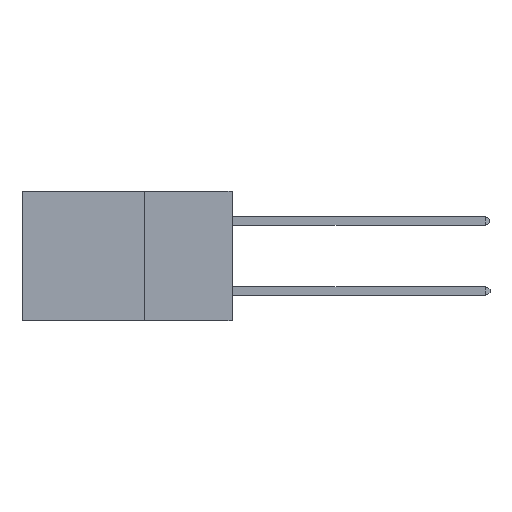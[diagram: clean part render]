
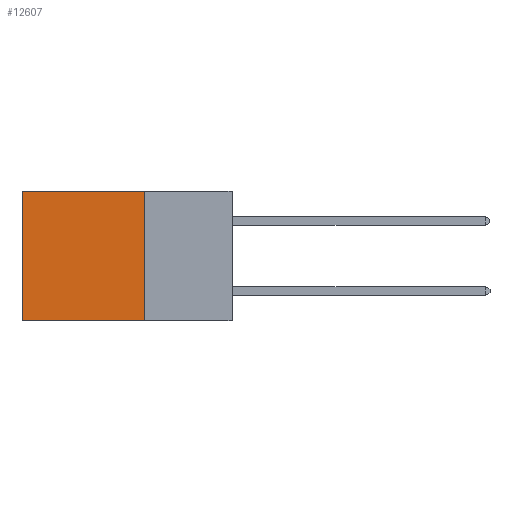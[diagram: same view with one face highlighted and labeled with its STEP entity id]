
A CAD part, left-side view. The second image highlights one B-rep face of the part: STEP entity #12607.
In plain terms, the highlighted planar face has unit normal (-1, 0, 0).
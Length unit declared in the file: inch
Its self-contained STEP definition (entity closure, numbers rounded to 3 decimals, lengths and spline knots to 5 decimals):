
#55 = ORIENTED_EDGE ( 'NONE', *, *, #5536, .T. ) ;
#754 = EDGE_CURVE ( 'NONE', #19839, #10343, #6532, .T. ) ;
#950 = CARTESIAN_POINT ( 'NONE',  ( 0.2875, 0.25, 0. ) ) ;
#1125 = DIRECTION ( 'NONE',  ( 0., 0., -1. ) ) ;
#1628 = VECTOR ( 'NONE', #1125, 39.37008 ) ;
#1685 = CARTESIAN_POINT ( 'NONE',  ( 0.2875, 0.6, 0. ) ) ;
#2611 = LINE ( 'NONE', #9584, #20841 ) ;
#2883 = VERTEX_POINT ( 'NONE', #950 ) ;
#3280 = ORIENTED_EDGE ( 'NONE', *, *, #20643, .F. ) ;
#3626 = PLANE ( 'NONE',  #17060 ) ;
#5319 = VECTOR ( 'NONE', #19799, 39.37008 ) ;
#5484 = DIRECTION ( 'NONE',  ( 1., 0., 0. ) ) ;
#5536 = EDGE_CURVE ( 'NONE', #2883, #19839, #2611, .T. ) ;
#6112 = DIRECTION ( 'NONE',  ( 0., 1., 0. ) ) ;
#6532 = LINE ( 'NONE', #6594, #1628 ) ;
#6594 = CARTESIAN_POINT ( 'NONE',  ( 0.2875, 0.6, 0. ) ) ;
#8834 = EDGE_CURVE ( 'NONE', #19460, #10343, #20507, .T. ) ;
#9584 = CARTESIAN_POINT ( 'NONE',  ( 0.2875, 0.25, 0. ) ) ;
#9641 = CARTESIAN_POINT ( 'NONE',  ( 0.2875, 0.25, -0.37 ) ) ;
#10343 = VERTEX_POINT ( 'NONE', #16460 ) ;
#11148 = VECTOR ( 'NONE', #6112, 39.37008 ) ;
#11332 = CARTESIAN_POINT ( 'NONE',  ( 0.2875, 0.25, -0.37 ) ) ;
#12607 = ADVANCED_FACE ( 'NONE', ( #19831 ), #3626, .F. ) ;
#14423 = CARTESIAN_POINT ( 'NONE',  ( 0.2875, 0.25, 0. ) ) ;
#14804 = DIRECTION ( 'NONE',  ( 0., 1., 0. ) ) ;
#15661 = LINE ( 'NONE', #14423, #5319 ) ;
#15690 = EDGE_LOOP ( 'NONE', ( #16634, #20914, #3280, #55 ) ) ;
#16460 = CARTESIAN_POINT ( 'NONE',  ( 0.2875, 0.6, -0.37 ) ) ;
#16634 = ORIENTED_EDGE ( 'NONE', *, *, #754, .T. ) ;
#17060 = AXIS2_PLACEMENT_3D ( 'NONE', #21072, #5484, #17709 ) ;
#17709 = DIRECTION ( 'NONE',  ( 0., 0., -1. ) ) ;
#19460 = VERTEX_POINT ( 'NONE', #9641 ) ;
#19799 = DIRECTION ( 'NONE',  ( 0., 0., -1. ) ) ;
#19831 = FACE_OUTER_BOUND ( 'NONE', #15690, .T. ) ;
#19839 = VERTEX_POINT ( 'NONE', #1685 ) ;
#20507 = LINE ( 'NONE', #11332, #11148 ) ;
#20643 = EDGE_CURVE ( 'NONE', #2883, #19460, #15661, .T. ) ;
#20841 = VECTOR ( 'NONE', #14804, 39.37008 ) ;
#20914 = ORIENTED_EDGE ( 'NONE', *, *, #8834, .F. ) ;
#21072 = CARTESIAN_POINT ( 'NONE',  ( 0.2875, 0.25, 0. ) ) ;
